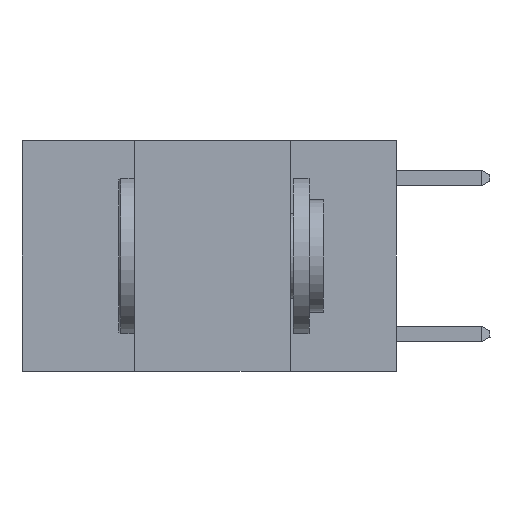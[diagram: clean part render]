
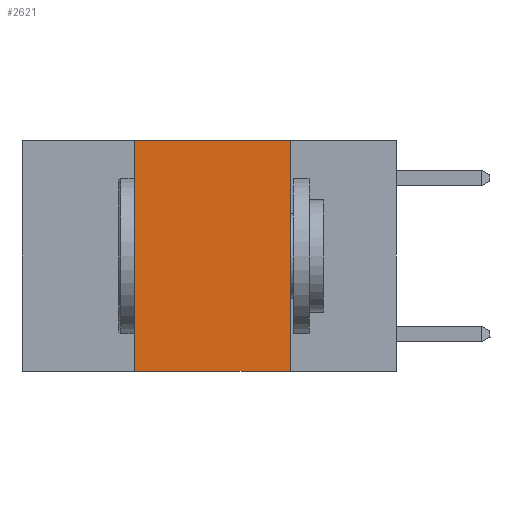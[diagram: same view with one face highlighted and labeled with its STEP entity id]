
A CAD part, left-side view. The second image highlights one B-rep face of the part: STEP entity #2621.
In plain terms, the highlighted planar face has unit normal (-1, 0, 0).
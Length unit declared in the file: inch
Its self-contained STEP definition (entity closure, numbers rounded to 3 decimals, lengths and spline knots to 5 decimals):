
#697 = CARTESIAN_POINT ( 'NONE',  ( 0., 0.42, -0.37 ) ) ;
#884 = AXIS2_PLACEMENT_3D ( 'NONE', #10822, #11802, #5815 ) ;
#922 = VECTOR ( 'NONE', #7887, 39.37008 ) ;
#1341 = LINE ( 'NONE', #8701, #8902 ) ;
#1496 = DIRECTION ( 'NONE',  ( 0., 0., -1. ) ) ;
#1647 = PLANE ( 'NONE',  #884 ) ;
#1691 = VERTEX_POINT ( 'NONE', #3210 ) ;
#2467 = DIRECTION ( 'NONE',  ( 0., 0., 1. ) ) ;
#2621 = ADVANCED_FACE ( 'NONE', ( #4992 ), #1647, .F. ) ;
#3210 = CARTESIAN_POINT ( 'NONE',  ( 0., 0.17, 0. ) ) ;
#3739 = EDGE_CURVE ( 'NONE', #10096, #1691, #11734, .T. ) ;
#4952 = DIRECTION ( 'NONE',  ( 0., -1., 0. ) ) ;
#4992 = FACE_OUTER_BOUND ( 'NONE', #9562, .T. ) ;
#5371 = ORIENTED_EDGE ( 'NONE', *, *, #10505, .F. ) ;
#5815 = DIRECTION ( 'NONE',  ( 0., 0., -1. ) ) ;
#6004 = CARTESIAN_POINT ( 'NONE',  ( 0., 0.6, -0.37 ) ) ;
#6219 = CARTESIAN_POINT ( 'NONE',  ( 0., 0.42, 0. ) ) ;
#6433 = LINE ( 'NONE', #6004, #8498 ) ;
#6458 = EDGE_CURVE ( 'NONE', #8882, #10096, #8980, .T. ) ;
#6528 = CARTESIAN_POINT ( 'NONE',  ( 0., 0.42, 0. ) ) ;
#6728 = EDGE_CURVE ( 'NONE', #8882, #7466, #6433, .T. ) ;
#7455 = CARTESIAN_POINT ( 'NONE',  ( 0., 0.17, -0.37 ) ) ;
#7466 = VERTEX_POINT ( 'NONE', #7455 ) ;
#7887 = DIRECTION ( 'NONE',  ( 0., -1., 0. ) ) ;
#8498 = VECTOR ( 'NONE', #4952, 39.37008 ) ;
#8701 = CARTESIAN_POINT ( 'NONE',  ( 0., 0.17, 0. ) ) ;
#8882 = VERTEX_POINT ( 'NONE', #697 ) ;
#8902 = VECTOR ( 'NONE', #1496, 39.37008 ) ;
#8980 = LINE ( 'NONE', #6528, #11287 ) ;
#9562 = EDGE_LOOP ( 'NONE', ( #5371, #12632, #11879, #11855 ) ) ;
#10096 = VERTEX_POINT ( 'NONE', #6219 ) ;
#10505 = EDGE_CURVE ( 'NONE', #1691, #7466, #1341, .T. ) ;
#10822 = CARTESIAN_POINT ( 'NONE',  ( 0., 0.6, 0. ) ) ;
#11287 = VECTOR ( 'NONE', #2467, 39.37008 ) ;
#11734 = LINE ( 'NONE', #11771, #922 ) ;
#11771 = CARTESIAN_POINT ( 'NONE',  ( 0., 0.6, 0. ) ) ;
#11802 = DIRECTION ( 'NONE',  ( 1., 0., 0. ) ) ;
#11855 = ORIENTED_EDGE ( 'NONE', *, *, #6728, .T. ) ;
#11879 = ORIENTED_EDGE ( 'NONE', *, *, #6458, .F. ) ;
#12632 = ORIENTED_EDGE ( 'NONE', *, *, #3739, .F. ) ;
